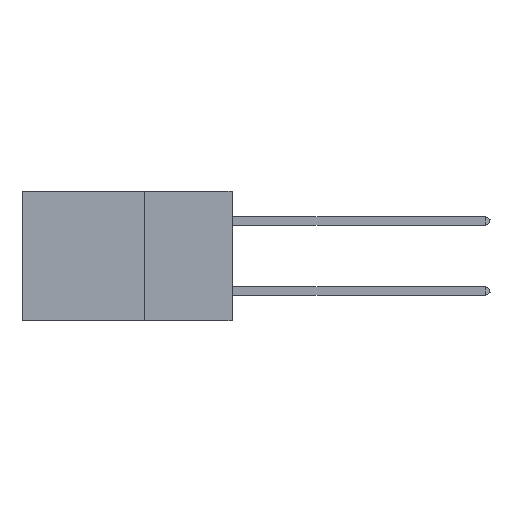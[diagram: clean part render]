
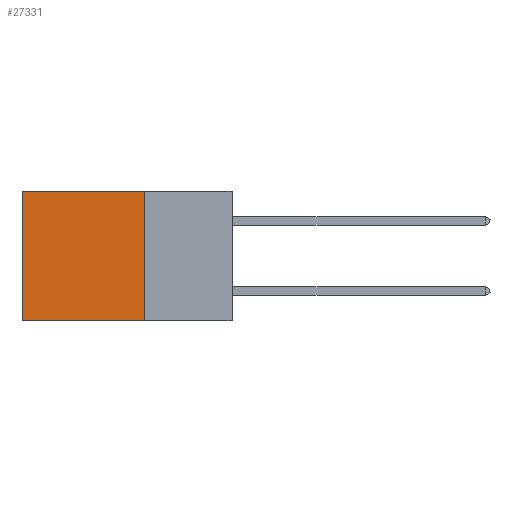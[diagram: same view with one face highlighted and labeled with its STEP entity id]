
A CAD part, left-side view. The second image highlights one B-rep face of the part: STEP entity #27331.
In plain terms, the highlighted planar face has unit normal (-1, 0, 0).
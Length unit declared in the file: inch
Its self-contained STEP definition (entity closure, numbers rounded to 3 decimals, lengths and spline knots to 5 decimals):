
#1245 = EDGE_CURVE ( 'NONE', #43842, #18054, #39876, .T. ) ;
#1616 = LINE ( 'NONE', #4869, #43291 ) ;
#4852 = VECTOR ( 'NONE', #8775, 39.37008 ) ;
#4869 = CARTESIAN_POINT ( 'NONE',  ( 0.2875, 0.25, 0. ) ) ;
#5055 = CARTESIAN_POINT ( 'NONE',  ( 0.2875, 0.25, -0.37 ) ) ;
#8530 = DIRECTION ( 'NONE',  ( 0., 0., -1. ) ) ;
#8775 = DIRECTION ( 'NONE',  ( 0., 1., 0. ) ) ;
#11290 = EDGE_CURVE ( 'NONE', #18054, #22232, #15155, .T. ) ;
#13454 = ORIENTED_EDGE ( 'NONE', *, *, #11290, .F. ) ;
#15155 = LINE ( 'NONE', #5055, #4852 ) ;
#17903 = EDGE_LOOP ( 'NONE', ( #37898, #13454, #44803, #45447 ) ) ;
#17944 = DIRECTION ( 'NONE',  ( 0., 0., -1. ) ) ;
#18054 = VERTEX_POINT ( 'NONE', #18244 ) ;
#18244 = CARTESIAN_POINT ( 'NONE',  ( 0.2875, 0.25, -0.37 ) ) ;
#18257 = CARTESIAN_POINT ( 'NONE',  ( 0.2875, 0.25, 0. ) ) ;
#18449 = CARTESIAN_POINT ( 'NONE',  ( 0.2875, 0.6, -0.37 ) ) ;
#22232 = VERTEX_POINT ( 'NONE', #18449 ) ;
#22649 = DIRECTION ( 'NONE',  ( 0., 0., -1. ) ) ;
#23113 = LINE ( 'NONE', #37021, #45909 ) ;
#23313 = VERTEX_POINT ( 'NONE', #27893 ) ;
#25717 = DIRECTION ( 'NONE',  ( 1., 0., 0. ) ) ;
#26921 = DIRECTION ( 'NONE',  ( 0., 1., 0. ) ) ;
#27331 = ADVANCED_FACE ( 'NONE', ( #31201 ), #28763, .F. ) ;
#27893 = CARTESIAN_POINT ( 'NONE',  ( 0.2875, 0.6, 0. ) ) ;
#28763 = PLANE ( 'NONE',  #39400 ) ;
#30194 = VECTOR ( 'NONE', #8530, 39.37008 ) ;
#30404 = CARTESIAN_POINT ( 'NONE',  ( 0.2875, 0.25, 0. ) ) ;
#31201 = FACE_OUTER_BOUND ( 'NONE', #17903, .T. ) ;
#34702 = CARTESIAN_POINT ( 'NONE',  ( 0.2875, 0.25, 0. ) ) ;
#37021 = CARTESIAN_POINT ( 'NONE',  ( 0.2875, 0.6, 0. ) ) ;
#37113 = EDGE_CURVE ( 'NONE', #43842, #23313, #1616, .T. ) ;
#37898 = ORIENTED_EDGE ( 'NONE', *, *, #40203, .T. ) ;
#39400 = AXIS2_PLACEMENT_3D ( 'NONE', #18257, #25717, #17944 ) ;
#39876 = LINE ( 'NONE', #30404, #30194 ) ;
#40203 = EDGE_CURVE ( 'NONE', #23313, #22232, #23113, .T. ) ;
#43291 = VECTOR ( 'NONE', #26921, 39.37008 ) ;
#43842 = VERTEX_POINT ( 'NONE', #34702 ) ;
#44803 = ORIENTED_EDGE ( 'NONE', *, *, #1245, .F. ) ;
#45447 = ORIENTED_EDGE ( 'NONE', *, *, #37113, .T. ) ;
#45909 = VECTOR ( 'NONE', #22649, 39.37008 ) ;
